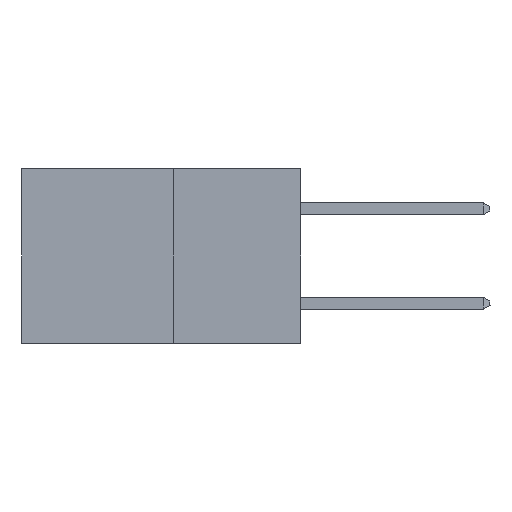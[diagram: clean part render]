
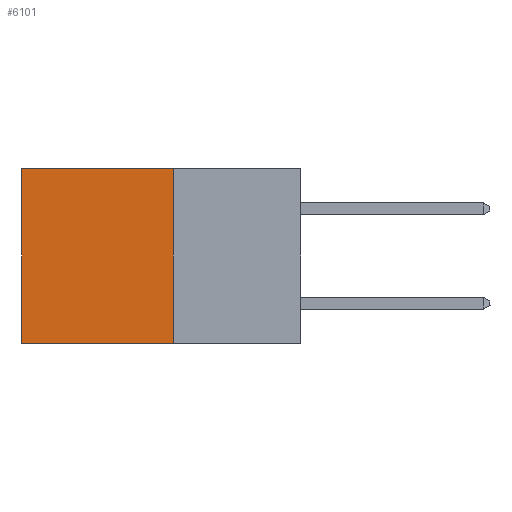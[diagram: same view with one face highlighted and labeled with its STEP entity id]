
A CAD part, left-side view. The second image highlights one B-rep face of the part: STEP entity #6101.
In plain terms, the highlighted planar face has unit normal (-1, 0, 0).
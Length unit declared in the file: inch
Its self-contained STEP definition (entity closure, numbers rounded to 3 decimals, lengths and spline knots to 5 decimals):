
#372 = EDGE_CURVE ( 'NONE', #985, #7501, #724, .T. ) ;
#724 = LINE ( 'NONE', #13743, #6840 ) ;
#985 = VERTEX_POINT ( 'NONE', #9185 ) ;
#1517 = EDGE_CURVE ( 'NONE', #13985, #985, #8653, .T. ) ;
#1956 = LINE ( 'NONE', #3246, #10799 ) ;
#2465 = ORIENTED_EDGE ( 'NONE', *, *, #1517, .F. ) ;
#2803 = EDGE_LOOP ( 'NONE', ( #5343, #8321, #2465, #14194 ) ) ;
#2831 = AXIS2_PLACEMENT_3D ( 'NONE', #11127, #4429, #12141 ) ;
#3024 = FACE_OUTER_BOUND ( 'NONE', #2803, .T. ) ;
#3246 = CARTESIAN_POINT ( 'NONE',  ( 0.277, 0.27, 0. ) ) ;
#4429 = DIRECTION ( 'NONE',  ( 1., 0., 0. ) ) ;
#5312 = VECTOR ( 'NONE', #12864, 39.37008 ) ;
#5343 = ORIENTED_EDGE ( 'NONE', *, *, #8130, .T. ) ;
#6101 = ADVANCED_FACE ( 'NONE', ( #3024 ), #13098, .F. ) ;
#6276 = CARTESIAN_POINT ( 'NONE',  ( 0.277, 0.59, -0.37 ) ) ;
#6830 = CARTESIAN_POINT ( 'NONE',  ( 0.277, 0.27, -0.37 ) ) ;
#6840 = VECTOR ( 'NONE', #11803, 39.37008 ) ;
#7501 = VERTEX_POINT ( 'NONE', #10008 ) ;
#8130 = EDGE_CURVE ( 'NONE', #14517, #7501, #11330, .T. ) ;
#8321 = ORIENTED_EDGE ( 'NONE', *, *, #372, .F. ) ;
#8619 = CARTESIAN_POINT ( 'NONE',  ( 0.277, 0.27, 0. ) ) ;
#8653 = LINE ( 'NONE', #6830, #5312 ) ;
#9185 = CARTESIAN_POINT ( 'NONE',  ( 0.277, 0.27, -0.37 ) ) ;
#10008 = CARTESIAN_POINT ( 'NONE',  ( 0.277, 0.59, -0.37 ) ) ;
#10053 = EDGE_CURVE ( 'NONE', #13985, #14517, #1956, .T. ) ;
#10799 = VECTOR ( 'NONE', #13202, 39.37008 ) ;
#11127 = CARTESIAN_POINT ( 'NONE',  ( 0.277, 0.27, -0.37 ) ) ;
#11330 = LINE ( 'NONE', #6276, #11646 ) ;
#11646 = VECTOR ( 'NONE', #12716, 39.37008 ) ;
#11803 = DIRECTION ( 'NONE',  ( 0., 1., 0. ) ) ;
#12141 = DIRECTION ( 'NONE',  ( 0., 0., -1. ) ) ;
#12716 = DIRECTION ( 'NONE',  ( 0., 0., -1. ) ) ;
#12864 = DIRECTION ( 'NONE',  ( 0., 0., -1. ) ) ;
#13098 = PLANE ( 'NONE',  #2831 ) ;
#13202 = DIRECTION ( 'NONE',  ( 0., 1., 0. ) ) ;
#13361 = CARTESIAN_POINT ( 'NONE',  ( 0.277, 0.59, 0. ) ) ;
#13743 = CARTESIAN_POINT ( 'NONE',  ( 0.277, 0.27, -0.37 ) ) ;
#13985 = VERTEX_POINT ( 'NONE', #8619 ) ;
#14194 = ORIENTED_EDGE ( 'NONE', *, *, #10053, .T. ) ;
#14517 = VERTEX_POINT ( 'NONE', #13361 ) ;
